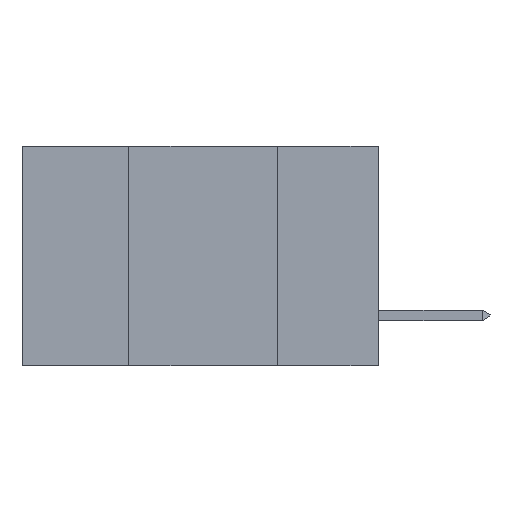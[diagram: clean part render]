
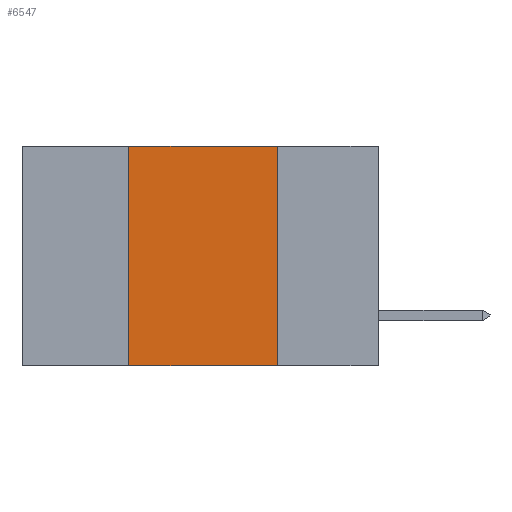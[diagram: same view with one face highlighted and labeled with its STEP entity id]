
A CAD part, left-side view. The second image highlights one B-rep face of the part: STEP entity #6547.
In plain terms, the highlighted planar face has unit normal (-1, 0, 0).
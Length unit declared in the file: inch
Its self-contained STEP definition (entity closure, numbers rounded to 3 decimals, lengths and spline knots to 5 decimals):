
#52 = VERTEX_POINT ( 'NONE', #5241 ) ;
#185 = DIRECTION ( 'NONE',  ( 0., -1., 0. ) ) ;
#230 = LINE ( 'NONE', #6735, #5918 ) ;
#511 = PLANE ( 'NONE',  #6751 ) ;
#534 = VERTEX_POINT ( 'NONE', #8945 ) ;
#570 = VERTEX_POINT ( 'NONE', #727 ) ;
#727 = CARTESIAN_POINT ( 'NONE',  ( 0., 0.42, 0. ) ) ;
#801 = LINE ( 'NONE', #7674, #5287 ) ;
#1021 = CARTESIAN_POINT ( 'NONE',  ( 0., 0.17, -0.37 ) ) ;
#1456 = EDGE_CURVE ( 'NONE', #52, #534, #2998, .T. ) ;
#1567 = EDGE_CURVE ( 'NONE', #570, #2313, #230, .T. ) ;
#1885 = ORIENTED_EDGE ( 'NONE', *, *, #1567, .F. ) ;
#2240 = DIRECTION ( 'NONE',  ( 0., 0., 1. ) ) ;
#2313 = VERTEX_POINT ( 'NONE', #2807 ) ;
#2683 = EDGE_CURVE ( 'NONE', #52, #570, #801, .T. ) ;
#2726 = FACE_OUTER_BOUND ( 'NONE', #6092, .T. ) ;
#2807 = CARTESIAN_POINT ( 'NONE',  ( 0., 0.17, 0. ) ) ;
#2998 = LINE ( 'NONE', #7928, #6638 ) ;
#3238 = EDGE_CURVE ( 'NONE', #2313, #534, #7331, .T. ) ;
#3241 = DIRECTION ( 'NONE',  ( 0., -1., 0. ) ) ;
#3245 = CARTESIAN_POINT ( 'NONE',  ( 0., 0.6, 0. ) ) ;
#3841 = DIRECTION ( 'NONE',  ( 0., 0., -1. ) ) ;
#5241 = CARTESIAN_POINT ( 'NONE',  ( 0., 0.42, -0.37 ) ) ;
#5249 = VECTOR ( 'NONE', #3841, 39.37008 ) ;
#5287 = VECTOR ( 'NONE', #2240, 39.37008 ) ;
#5352 = ORIENTED_EDGE ( 'NONE', *, *, #1456, .T. ) ;
#5918 = VECTOR ( 'NONE', #3241, 39.37008 ) ;
#6092 = EDGE_LOOP ( 'NONE', ( #8057, #1885, #6765, #5352 ) ) ;
#6547 = ADVANCED_FACE ( 'NONE', ( #2726 ), #511, .F. ) ;
#6638 = VECTOR ( 'NONE', #185, 39.37008 ) ;
#6735 = CARTESIAN_POINT ( 'NONE',  ( 0., 0.6, 0. ) ) ;
#6751 = AXIS2_PLACEMENT_3D ( 'NONE', #3245, #7522, #8282 ) ;
#6765 = ORIENTED_EDGE ( 'NONE', *, *, #2683, .F. ) ;
#7331 = LINE ( 'NONE', #1021, #5249 ) ;
#7522 = DIRECTION ( 'NONE',  ( 1., 0., 0. ) ) ;
#7674 = CARTESIAN_POINT ( 'NONE',  ( 0., 0.42, -0.37 ) ) ;
#7928 = CARTESIAN_POINT ( 'NONE',  ( 0., 0.6, -0.37 ) ) ;
#8057 = ORIENTED_EDGE ( 'NONE', *, *, #3238, .F. ) ;
#8282 = DIRECTION ( 'NONE',  ( 0., 0., -1. ) ) ;
#8945 = CARTESIAN_POINT ( 'NONE',  ( 0., 0.17, -0.37 ) ) ;
